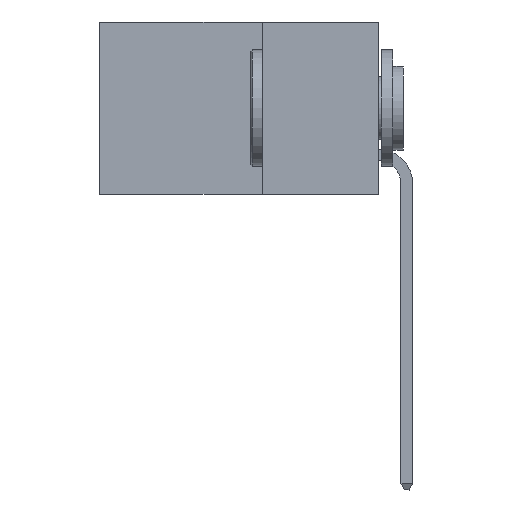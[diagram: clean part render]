
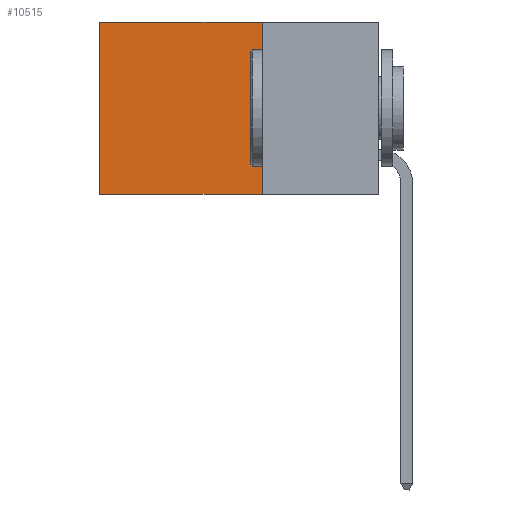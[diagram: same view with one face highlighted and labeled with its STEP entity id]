
A CAD part, left-side view. The second image highlights one B-rep face of the part: STEP entity #10515.
In plain terms, the highlighted planar face has unit normal (-1, 0, 0).
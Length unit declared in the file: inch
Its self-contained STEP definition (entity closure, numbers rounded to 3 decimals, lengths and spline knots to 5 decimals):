
#540 = CARTESIAN_POINT ( 'NONE',  ( 0.298, 0.25, 0. ) ) ;
#579 = EDGE_CURVE ( 'NONE', #31337, #5765, #826, .T. ) ;
#805 = ORIENTED_EDGE ( 'NONE', *, *, #15910, .T. ) ;
#826 = LINE ( 'NONE', #15132, #23938 ) ;
#1878 = ORIENTED_EDGE ( 'NONE', *, *, #23869, .T. ) ;
#2384 = EDGE_LOOP ( 'NONE', ( #805, #23479, #21268, #1878 ) ) ;
#2652 = PLANE ( 'NONE',  #30237 ) ;
#3781 = VERTEX_POINT ( 'NONE', #22763 ) ;
#5765 = VERTEX_POINT ( 'NONE', #24008 ) ;
#6511 = DIRECTION ( 'NONE',  ( 0., 0., -1. ) ) ;
#7599 = DIRECTION ( 'NONE',  ( 0., 0., -1. ) ) ;
#7888 = FACE_OUTER_BOUND ( 'NONE', #2384, .T. ) ;
#10171 = CARTESIAN_POINT ( 'NONE',  ( 0.298, 0.25, -0.37 ) ) ;
#10515 = ADVANCED_FACE ( 'NONE', ( #7888 ), #2652, .F. ) ;
#14014 = CARTESIAN_POINT ( 'NONE',  ( 0.298, 0.25, 0. ) ) ;
#14095 = CARTESIAN_POINT ( 'NONE',  ( 0.298, 0.25, 0. ) ) ;
#15132 = CARTESIAN_POINT ( 'NONE',  ( 0.298, 0.25, -0.37 ) ) ;
#15910 = EDGE_CURVE ( 'NONE', #3781, #5765, #26786, .T. ) ;
#17157 = DIRECTION ( 'NONE',  ( 1., 0., 0. ) ) ;
#17566 = DIRECTION ( 'NONE',  ( 0., 1., 0. ) ) ;
#18682 = DIRECTION ( 'NONE',  ( 0., 1., 0. ) ) ;
#19402 = CARTESIAN_POINT ( 'NONE',  ( 0.298, 0.25, 0. ) ) ;
#20622 = DIRECTION ( 'NONE',  ( 0., 0., -1. ) ) ;
#21268 = ORIENTED_EDGE ( 'NONE', *, *, #29745, .F. ) ;
#22763 = CARTESIAN_POINT ( 'NONE',  ( 0.298, 0.6, 0. ) ) ;
#23400 = VECTOR ( 'NONE', #20622, 39.37008 ) ;
#23479 = ORIENTED_EDGE ( 'NONE', *, *, #579, .F. ) ;
#23869 = EDGE_CURVE ( 'NONE', #30847, #3781, #26501, .T. ) ;
#23938 = VECTOR ( 'NONE', #17566, 39.37008 ) ;
#24008 = CARTESIAN_POINT ( 'NONE',  ( 0.298, 0.6, -0.37 ) ) ;
#25586 = LINE ( 'NONE', #14014, #30907 ) ;
#26501 = LINE ( 'NONE', #14095, #28395 ) ;
#26786 = LINE ( 'NONE', #27755, #23400 ) ;
#27755 = CARTESIAN_POINT ( 'NONE',  ( 0.298, 0.6, 0. ) ) ;
#28395 = VECTOR ( 'NONE', #18682, 39.37008 ) ;
#29745 = EDGE_CURVE ( 'NONE', #30847, #31337, #25586, .T. ) ;
#30237 = AXIS2_PLACEMENT_3D ( 'NONE', #19402, #17157, #7599 ) ;
#30847 = VERTEX_POINT ( 'NONE', #540 ) ;
#30907 = VECTOR ( 'NONE', #6511, 39.37008 ) ;
#31337 = VERTEX_POINT ( 'NONE', #10171 ) ;
